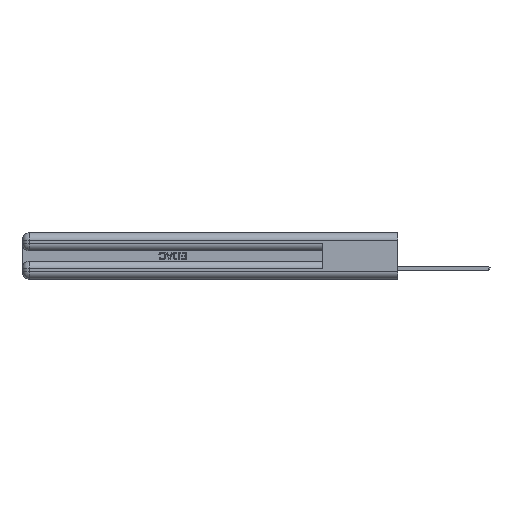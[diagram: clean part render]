
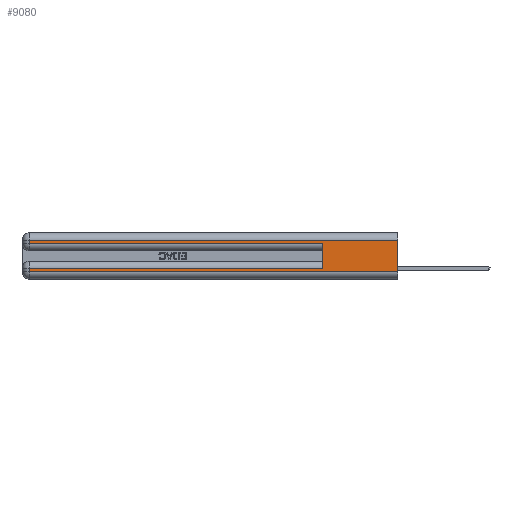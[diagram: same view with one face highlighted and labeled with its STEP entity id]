
A CAD part, left-side view. The second image highlights one B-rep face of the part: STEP entity #9080.
In plain terms, the highlighted planar face has unit normal (-1, 0, 0).
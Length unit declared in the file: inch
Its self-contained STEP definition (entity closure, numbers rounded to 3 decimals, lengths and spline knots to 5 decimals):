
#778 = CARTESIAN_POINT ( 'NONE',  ( 0., 0.6, 0.145 ) ) ;
#3864 = VERTEX_POINT ( 'NONE', #42663 ) ;
#3956 = EDGE_LOOP ( 'NONE', ( #33915, #48766, #17194, #15602, #41119, #16935, #34184, #17984 ) ) ;
#4647 = CARTESIAN_POINT ( 'NONE',  ( 0., 2.94, 0.06 ) ) ;
#6195 = DIRECTION ( 'NONE',  ( 0., 0., -1. ) ) ;
#6486 = LINE ( 'NONE', #12684, #7754 ) ;
#7370 = LINE ( 'NONE', #778, #28127 ) ;
#7754 = VECTOR ( 'NONE', #13029, 39.37008 ) ;
#8371 = CARTESIAN_POINT ( 'NONE',  ( 0., 0., 0.31 ) ) ;
#9080 = ADVANCED_FACE ( 'NONE', ( #40137 ), #37482, .F. ) ;
#9822 = CARTESIAN_POINT ( 'NONE',  ( 0., 0., 0.37 ) ) ;
#12684 = CARTESIAN_POINT ( 'NONE',  ( 0., 0., 0.06 ) ) ;
#13029 = DIRECTION ( 'NONE',  ( 0., -1., 0. ) ) ;
#14539 = EDGE_CURVE ( 'NONE', #31488, #27480, #44477, .T. ) ;
#14663 = VECTOR ( 'NONE', #24651, 39.37008 ) ;
#15602 = ORIENTED_EDGE ( 'NONE', *, *, #44339, .T. ) ;
#16935 = ORIENTED_EDGE ( 'NONE', *, *, #38532, .T. ) ;
#16991 = EDGE_CURVE ( 'NONE', #42885, #27480, #6486, .T. ) ;
#17194 = ORIENTED_EDGE ( 'NONE', *, *, #41066, .T. ) ;
#17917 = CARTESIAN_POINT ( 'NONE',  ( 0., 0., 0.085 ) ) ;
#17984 = ORIENTED_EDGE ( 'NONE', *, *, #16991, .T. ) ;
#18024 = DIRECTION ( 'NONE',  ( 1., 0., 0. ) ) ;
#18611 = VERTEX_POINT ( 'NONE', #49074 ) ;
#19010 = EDGE_CURVE ( 'NONE', #31488, #3864, #39948, .T. ) ;
#20136 = EDGE_CURVE ( 'NONE', #27469, #42885, #47332, .T. ) ;
#20355 = VECTOR ( 'NONE', #30079, 39.37008 ) ;
#21190 = CARTESIAN_POINT ( 'NONE',  ( 0., 2.94, 0.285 ) ) ;
#22041 = DIRECTION ( 'NONE',  ( 0., 0., -1. ) ) ;
#22108 = CARTESIAN_POINT ( 'NONE',  ( 0., 0., 0.31 ) ) ;
#22920 = VECTOR ( 'NONE', #48665, 39.37008 ) ;
#23614 = CARTESIAN_POINT ( 'NONE',  ( 0., 2.94, 0.085 ) ) ;
#24651 = DIRECTION ( 'NONE',  ( 0., 0., -1. ) ) ;
#27469 = VERTEX_POINT ( 'NONE', #23614 ) ;
#27480 = VERTEX_POINT ( 'NONE', #35407 ) ;
#28127 = VECTOR ( 'NONE', #49127, 39.37008 ) ;
#29105 = VERTEX_POINT ( 'NONE', #21190 ) ;
#29136 = AXIS2_PLACEMENT_3D ( 'NONE', #9822, #18024, #22041 ) ;
#30076 = LINE ( 'NONE', #17917, #49572 ) ;
#30079 = DIRECTION ( 'NONE',  ( 0., 0., -1. ) ) ;
#31488 = VERTEX_POINT ( 'NONE', #22108 ) ;
#33315 = VERTEX_POINT ( 'NONE', #50836 ) ;
#33915 = ORIENTED_EDGE ( 'NONE', *, *, #14539, .F. ) ;
#33995 = CARTESIAN_POINT ( 'NONE',  ( 0., 0., 0.37 ) ) ;
#34184 = ORIENTED_EDGE ( 'NONE', *, *, #20136, .T. ) ;
#35407 = CARTESIAN_POINT ( 'NONE',  ( 0., 0., 0.06 ) ) ;
#35615 = CARTESIAN_POINT ( 'NONE',  ( 0., 2.94, 0.37 ) ) ;
#37482 = PLANE ( 'NONE',  #29136 ) ;
#38532 = EDGE_CURVE ( 'NONE', #33315, #27469, #30076, .T. ) ;
#39187 = EDGE_CURVE ( 'NONE', #33315, #18611, #7370, .T. ) ;
#39948 = LINE ( 'NONE', #8371, #22920 ) ;
#40137 = FACE_OUTER_BOUND ( 'NONE', #3956, .T. ) ;
#41066 = EDGE_CURVE ( 'NONE', #3864, #29105, #47419, .T. ) ;
#41119 = ORIENTED_EDGE ( 'NONE', *, *, #39187, .F. ) ;
#41847 = DIRECTION ( 'NONE',  ( 0., -1., 0. ) ) ;
#42116 = CARTESIAN_POINT ( 'NONE',  ( 0., 2.94, 0.37 ) ) ;
#42663 = CARTESIAN_POINT ( 'NONE',  ( 0., 2.94, 0.31 ) ) ;
#42885 = VERTEX_POINT ( 'NONE', #4647 ) ;
#44339 = EDGE_CURVE ( 'NONE', #29105, #18611, #44967, .T. ) ;
#44477 = LINE ( 'NONE', #33995, #48274 ) ;
#44967 = LINE ( 'NONE', #49724, #48131 ) ;
#47332 = LINE ( 'NONE', #35615, #14663 ) ;
#47419 = LINE ( 'NONE', #42116, #20355 ) ;
#48131 = VECTOR ( 'NONE', #41847, 39.37008 ) ;
#48274 = VECTOR ( 'NONE', #6195, 39.37008 ) ;
#48665 = DIRECTION ( 'NONE',  ( 0., 1., 0. ) ) ;
#48766 = ORIENTED_EDGE ( 'NONE', *, *, #19010, .T. ) ;
#49074 = CARTESIAN_POINT ( 'NONE',  ( 0., 0.6, 0.285 ) ) ;
#49127 = DIRECTION ( 'NONE',  ( 0., 0., 1. ) ) ;
#49572 = VECTOR ( 'NONE', #49842, 39.37008 ) ;
#49724 = CARTESIAN_POINT ( 'NONE',  ( 0., 0., 0.285 ) ) ;
#49842 = DIRECTION ( 'NONE',  ( 0., 1., 0. ) ) ;
#50836 = CARTESIAN_POINT ( 'NONE',  ( 0., 0.6, 0.085 ) ) ;
